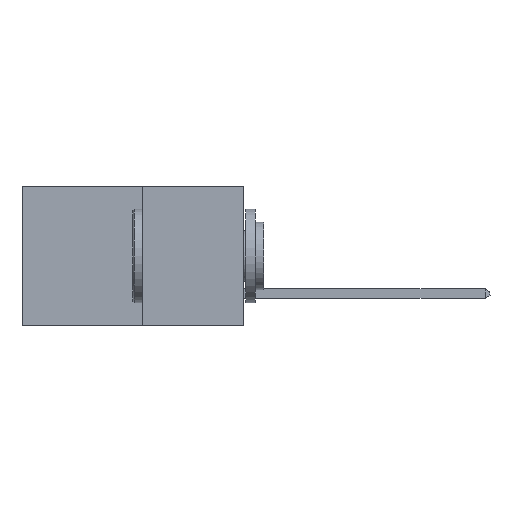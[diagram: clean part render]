
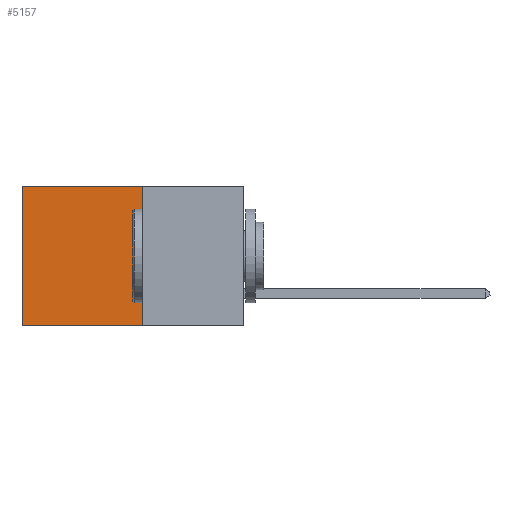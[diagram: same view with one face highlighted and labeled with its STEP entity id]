
A CAD part, left-side view. The second image highlights one B-rep face of the part: STEP entity #5157.
In plain terms, the highlighted planar face has unit normal (-1, 0, 0).
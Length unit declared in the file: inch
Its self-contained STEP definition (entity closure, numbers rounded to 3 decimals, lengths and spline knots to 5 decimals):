
#264 = VECTOR ( 'NONE', #2320, 39.37008 ) ;
#550 = LINE ( 'NONE', #6476, #264 ) ;
#781 = ORIENTED_EDGE ( 'NONE', *, *, #2051, .F. ) ;
#919 = VERTEX_POINT ( 'NONE', #6647 ) ;
#954 = EDGE_CURVE ( 'NONE', #5152, #8061, #2363, .T. ) ;
#976 = DIRECTION ( 'NONE',  ( 0., 0., -1. ) ) ;
#1073 = DIRECTION ( 'NONE',  ( 1., 0., 0. ) ) ;
#1148 = PLANE ( 'NONE',  #4150 ) ;
#1312 = CARTESIAN_POINT ( 'NONE',  ( 0.277, 0.27, 0. ) ) ;
#1569 = CARTESIAN_POINT ( 'NONE',  ( 0.277, 0.27, -0.37 ) ) ;
#2051 = EDGE_CURVE ( 'NONE', #8061, #6574, #550, .T. ) ;
#2123 = DIRECTION ( 'NONE',  ( 0., 0., -1. ) ) ;
#2190 = LINE ( 'NONE', #7159, #6629 ) ;
#2320 = DIRECTION ( 'NONE',  ( 0., 1., 0. ) ) ;
#2363 = LINE ( 'NONE', #4447, #6286 ) ;
#2435 = CARTESIAN_POINT ( 'NONE',  ( 0.277, 0.59, -0.37 ) ) ;
#3068 = DIRECTION ( 'NONE',  ( 0., 0., -1. ) ) ;
#3200 = EDGE_CURVE ( 'NONE', #919, #6574, #2190, .T. ) ;
#4083 = CARTESIAN_POINT ( 'NONE',  ( 0.277, 0.27, -0.37 ) ) ;
#4104 = DIRECTION ( 'NONE',  ( 0., 1., 0. ) ) ;
#4150 = AXIS2_PLACEMENT_3D ( 'NONE', #1569, #1073, #976 ) ;
#4447 = CARTESIAN_POINT ( 'NONE',  ( 0.277, 0.27, -0.37 ) ) ;
#4529 = ORIENTED_EDGE ( 'NONE', *, *, #10036, .T. ) ;
#5032 = FACE_OUTER_BOUND ( 'NONE', #8277, .T. ) ;
#5152 = VERTEX_POINT ( 'NONE', #1312 ) ;
#5157 = ADVANCED_FACE ( 'NONE', ( #5032 ), #1148, .F. ) ;
#6113 = ORIENTED_EDGE ( 'NONE', *, *, #954, .F. ) ;
#6223 = ORIENTED_EDGE ( 'NONE', *, *, #3200, .T. ) ;
#6286 = VECTOR ( 'NONE', #2123, 39.37008 ) ;
#6476 = CARTESIAN_POINT ( 'NONE',  ( 0.277, 0.27, -0.37 ) ) ;
#6574 = VERTEX_POINT ( 'NONE', #2435 ) ;
#6629 = VECTOR ( 'NONE', #3068, 39.37008 ) ;
#6647 = CARTESIAN_POINT ( 'NONE',  ( 0.277, 0.59, 0. ) ) ;
#6671 = LINE ( 'NONE', #10501, #9534 ) ;
#7159 = CARTESIAN_POINT ( 'NONE',  ( 0.277, 0.59, -0.37 ) ) ;
#8061 = VERTEX_POINT ( 'NONE', #4083 ) ;
#8277 = EDGE_LOOP ( 'NONE', ( #6223, #781, #6113, #4529 ) ) ;
#9534 = VECTOR ( 'NONE', #4104, 39.37008 ) ;
#10036 = EDGE_CURVE ( 'NONE', #5152, #919, #6671, .T. ) ;
#10501 = CARTESIAN_POINT ( 'NONE',  ( 0.277, 0.27, 0. ) ) ;
